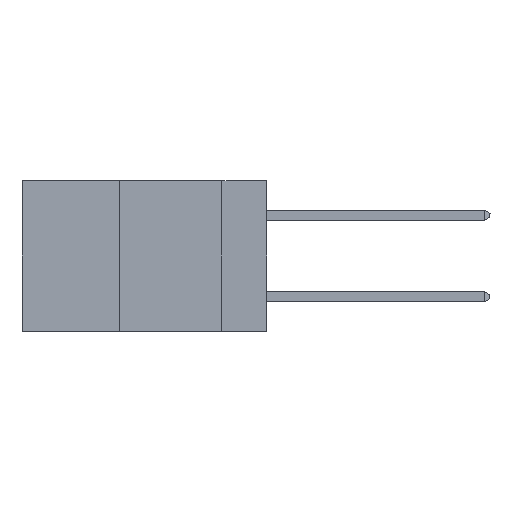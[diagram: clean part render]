
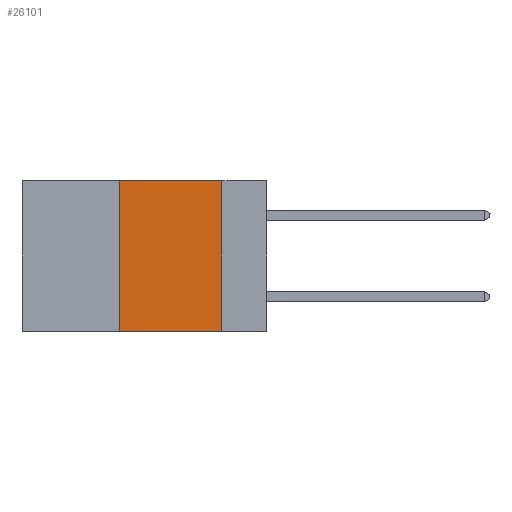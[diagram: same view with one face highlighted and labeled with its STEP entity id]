
A CAD part, left-side view. The second image highlights one B-rep face of the part: STEP entity #26101.
In plain terms, the highlighted planar face has unit normal (-1, 0, 0).
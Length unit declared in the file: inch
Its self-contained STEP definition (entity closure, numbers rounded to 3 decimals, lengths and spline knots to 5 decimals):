
#460 = FACE_OUTER_BOUND ( 'NONE', #4599, .T. ) ;
#1069 = VERTEX_POINT ( 'NONE', #24765 ) ;
#1632 = DIRECTION ( 'NONE',  ( 0., 0., -1. ) ) ;
#2975 = DIRECTION ( 'NONE',  ( 0., -1., 0. ) ) ;
#3076 = EDGE_CURVE ( 'NONE', #29102, #1069, #29304, .T. ) ;
#3810 = CARTESIAN_POINT ( 'NONE',  ( 0., 0.6, 0. ) ) ;
#4599 = EDGE_LOOP ( 'NONE', ( #16127, #16313, #16398, #16643 ) ) ;
#6369 = CARTESIAN_POINT ( 'NONE',  ( 0., 0.36, 0. ) ) ;
#6616 = VERTEX_POINT ( 'NONE', #11378 ) ;
#7016 = VECTOR ( 'NONE', #11212, 39.37008 ) ;
#8807 = EDGE_CURVE ( 'NONE', #6616, #29102, #15386, .T. ) ;
#8813 = CARTESIAN_POINT ( 'NONE',  ( 0., 0.6, 0. ) ) ;
#9012 = VECTOR ( 'NONE', #25105, 39.37008 ) ;
#10404 = AXIS2_PLACEMENT_3D ( 'NONE', #8813, #16044, #1632 ) ;
#11162 = EDGE_CURVE ( 'NONE', #21007, #6616, #25776, .T. ) ;
#11211 = PLANE ( 'NONE',  #10404 ) ;
#11212 = DIRECTION ( 'NONE',  ( 0., 0., 1. ) ) ;
#11378 = CARTESIAN_POINT ( 'NONE',  ( 0., 0.36, 0. ) ) ;
#13530 = VECTOR ( 'NONE', #2975, 39.37008 ) ;
#15386 = LINE ( 'NONE', #3810, #9012 ) ;
#15458 = CARTESIAN_POINT ( 'NONE',  ( 0., 0.11, 0. ) ) ;
#16044 = DIRECTION ( 'NONE',  ( 1., 0., 0. ) ) ;
#16127 = ORIENTED_EDGE ( 'NONE', *, *, #3076, .F. ) ;
#16313 = ORIENTED_EDGE ( 'NONE', *, *, #8807, .F. ) ;
#16398 = ORIENTED_EDGE ( 'NONE', *, *, #11162, .F. ) ;
#16643 = ORIENTED_EDGE ( 'NONE', *, *, #28312, .T. ) ;
#17162 = CARTESIAN_POINT ( 'NONE',  ( 0., 0.6, -0.37 ) ) ;
#19790 = LINE ( 'NONE', #17162, #13530 ) ;
#21007 = VERTEX_POINT ( 'NONE', #21821 ) ;
#21821 = CARTESIAN_POINT ( 'NONE',  ( 0., 0.36, -0.37 ) ) ;
#23219 = VECTOR ( 'NONE', #26928, 39.37008 ) ;
#24765 = CARTESIAN_POINT ( 'NONE',  ( 0., 0.11, -0.37 ) ) ;
#25105 = DIRECTION ( 'NONE',  ( 0., -1., 0. ) ) ;
#25776 = LINE ( 'NONE', #6369, #7016 ) ;
#26101 = ADVANCED_FACE ( 'NONE', ( #460 ), #11211, .F. ) ;
#26928 = DIRECTION ( 'NONE',  ( 0., 0., -1. ) ) ;
#27344 = CARTESIAN_POINT ( 'NONE',  ( 0., 0.11, 0. ) ) ;
#28312 = EDGE_CURVE ( 'NONE', #21007, #1069, #19790, .T. ) ;
#29102 = VERTEX_POINT ( 'NONE', #27344 ) ;
#29304 = LINE ( 'NONE', #15458, #23219 ) ;
